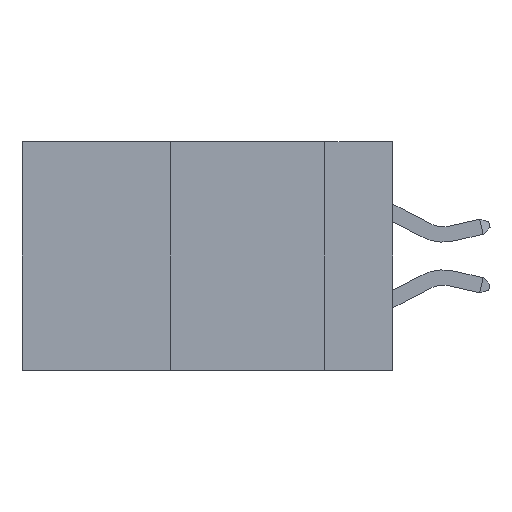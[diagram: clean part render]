
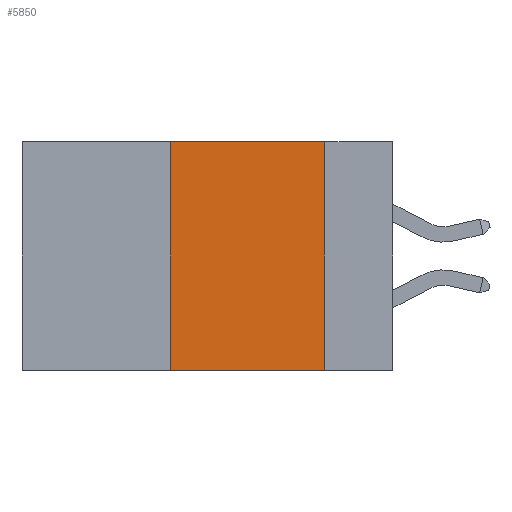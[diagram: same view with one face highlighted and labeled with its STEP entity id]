
A CAD part, left-side view. The second image highlights one B-rep face of the part: STEP entity #5850.
In plain terms, the highlighted planar face has unit normal (-1, 0, 0).
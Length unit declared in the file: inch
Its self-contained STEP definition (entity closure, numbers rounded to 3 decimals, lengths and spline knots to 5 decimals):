
#313 = LINE ( 'NONE', #16548, #13337 ) ;
#1912 = ORIENTED_EDGE ( 'NONE', *, *, #4376, .F. ) ;
#2658 = ORIENTED_EDGE ( 'NONE', *, *, #7858, .F. ) ;
#2698 = VECTOR ( 'NONE', #4855, 39.37008 ) ;
#3175 = CARTESIAN_POINT ( 'NONE',  ( 0., 0.6, -0.37 ) ) ;
#3261 = CARTESIAN_POINT ( 'NONE',  ( 0., 0.36, 0. ) ) ;
#3411 = ORIENTED_EDGE ( 'NONE', *, *, #14388, .F. ) ;
#3777 = ORIENTED_EDGE ( 'NONE', *, *, #4895, .T. ) ;
#3791 = PLANE ( 'NONE',  #12067 ) ;
#4293 = VERTEX_POINT ( 'NONE', #8360 ) ;
#4376 = EDGE_CURVE ( 'NONE', #4293, #17418, #313, .T. ) ;
#4855 = DIRECTION ( 'NONE',  ( 0., -1., 0. ) ) ;
#4895 = EDGE_CURVE ( 'NONE', #16357, #17418, #15153, .T. ) ;
#4946 = DIRECTION ( 'NONE',  ( 0., 0., 1. ) ) ;
#5323 = DIRECTION ( 'NONE',  ( 0., 0., -1. ) ) ;
#5850 = ADVANCED_FACE ( 'NONE', ( #14121 ), #3791, .F. ) ;
#7474 = CARTESIAN_POINT ( 'NONE',  ( 0., 0.11, -0.37 ) ) ;
#7858 = EDGE_CURVE ( 'NONE', #17500, #4293, #9250, .T. ) ;
#8360 = CARTESIAN_POINT ( 'NONE',  ( 0., 0.11, 0. ) ) ;
#8713 = CARTESIAN_POINT ( 'NONE',  ( 0., 0.6, 0. ) ) ;
#9250 = LINE ( 'NONE', #19131, #13052 ) ;
#9676 = EDGE_LOOP ( 'NONE', ( #1912, #2658, #3411, #3777 ) ) ;
#10356 = DIRECTION ( 'NONE',  ( 0., 0., -1. ) ) ;
#11181 = CARTESIAN_POINT ( 'NONE',  ( 0., 0.36, -0.37 ) ) ;
#12067 = AXIS2_PLACEMENT_3D ( 'NONE', #8713, #19855, #10356 ) ;
#13052 = VECTOR ( 'NONE', #14542, 39.37008 ) ;
#13337 = VECTOR ( 'NONE', #5323, 39.37008 ) ;
#14121 = FACE_OUTER_BOUND ( 'NONE', #9676, .T. ) ;
#14388 = EDGE_CURVE ( 'NONE', #16357, #17500, #20140, .T. ) ;
#14542 = DIRECTION ( 'NONE',  ( 0., -1., 0. ) ) ;
#15153 = LINE ( 'NONE', #3175, #2698 ) ;
#16357 = VERTEX_POINT ( 'NONE', #11181 ) ;
#16548 = CARTESIAN_POINT ( 'NONE',  ( 0., 0.11, 0. ) ) ;
#17260 = CARTESIAN_POINT ( 'NONE',  ( 0., 0.36, 0. ) ) ;
#17418 = VERTEX_POINT ( 'NONE', #7474 ) ;
#17500 = VERTEX_POINT ( 'NONE', #17260 ) ;
#19131 = CARTESIAN_POINT ( 'NONE',  ( 0., 0.6, 0. ) ) ;
#19668 = VECTOR ( 'NONE', #4946, 39.37008 ) ;
#19855 = DIRECTION ( 'NONE',  ( 1., 0., 0. ) ) ;
#20140 = LINE ( 'NONE', #3261, #19668 ) ;
